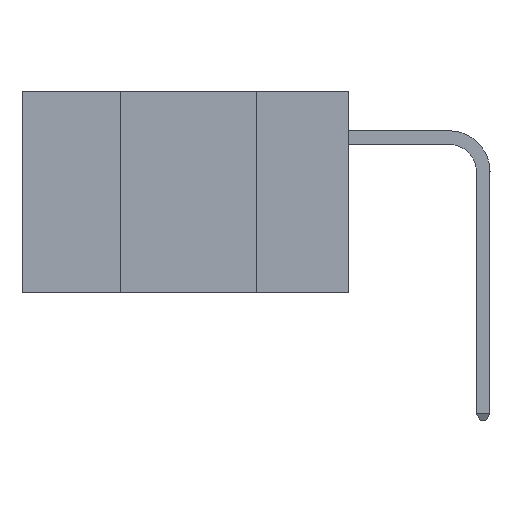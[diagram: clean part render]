
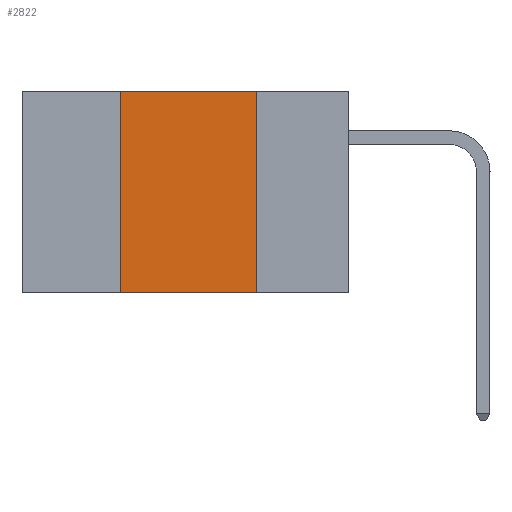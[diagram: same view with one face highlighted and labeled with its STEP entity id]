
A CAD part, left-side view. The second image highlights one B-rep face of the part: STEP entity #2822.
In plain terms, the highlighted planar face has unit normal (-1, 0, 0).
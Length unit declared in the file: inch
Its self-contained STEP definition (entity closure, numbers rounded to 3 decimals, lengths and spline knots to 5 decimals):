
#2822 = ADVANCED_FACE ( 'NONE', ( #23863 ), #23248, .F. ) ;
#2836 = DIRECTION ( 'NONE',  ( 0., 0., 1. ) ) ;
#5013 = AXIS2_PLACEMENT_3D ( 'NONE', #9218, #9372, #37027 ) ;
#6765 = CARTESIAN_POINT ( 'NONE',  ( 0., 0.42, 0. ) ) ;
#6784 = VECTOR ( 'NONE', #17891, 39.37008 ) ;
#8238 = VECTOR ( 'NONE', #37631, 39.37008 ) ;
#9218 = CARTESIAN_POINT ( 'NONE',  ( 0., 0.6, 0. ) ) ;
#9314 = LINE ( 'NONE', #23564, #8238 ) ;
#9372 = DIRECTION ( 'NONE',  ( 1., 0., 0. ) ) ;
#11196 = VERTEX_POINT ( 'NONE', #6765 ) ;
#12032 = ORIENTED_EDGE ( 'NONE', *, *, #25710, .F. ) ;
#12527 = EDGE_LOOP ( 'NONE', ( #12032, #18348, #21887, #29195 ) ) ;
#13264 = LINE ( 'NONE', #14585, #6784 ) ;
#14585 = CARTESIAN_POINT ( 'NONE',  ( 0., 0.6, 0. ) ) ;
#15386 = CARTESIAN_POINT ( 'NONE',  ( 0., 0.17, 0. ) ) ;
#16108 = CARTESIAN_POINT ( 'NONE',  ( 0., 0.42, 0. ) ) ;
#17497 = CARTESIAN_POINT ( 'NONE',  ( 0., 0.17, -0.37 ) ) ;
#17580 = LINE ( 'NONE', #16108, #38701 ) ;
#17891 = DIRECTION ( 'NONE',  ( 0., -1., 0. ) ) ;
#18348 = ORIENTED_EDGE ( 'NONE', *, *, #38684, .F. ) ;
#20844 = VERTEX_POINT ( 'NONE', #30768 ) ;
#21887 = ORIENTED_EDGE ( 'NONE', *, *, #38422, .F. ) ;
#23248 = PLANE ( 'NONE',  #5013 ) ;
#23564 = CARTESIAN_POINT ( 'NONE',  ( 0., 0.17, 0. ) ) ;
#23863 = FACE_OUTER_BOUND ( 'NONE', #12527, .T. ) ;
#25710 = EDGE_CURVE ( 'NONE', #32969, #40921, #9314, .T. ) ;
#26568 = LINE ( 'NONE', #42383, #39487 ) ;
#29195 = ORIENTED_EDGE ( 'NONE', *, *, #30340, .T. ) ;
#30340 = EDGE_CURVE ( 'NONE', #20844, #40921, #26568, .T. ) ;
#30768 = CARTESIAN_POINT ( 'NONE',  ( 0., 0.42, -0.37 ) ) ;
#32969 = VERTEX_POINT ( 'NONE', #15386 ) ;
#37027 = DIRECTION ( 'NONE',  ( 0., 0., -1. ) ) ;
#37631 = DIRECTION ( 'NONE',  ( 0., 0., -1. ) ) ;
#38422 = EDGE_CURVE ( 'NONE', #20844, #11196, #17580, .T. ) ;
#38684 = EDGE_CURVE ( 'NONE', #11196, #32969, #13264, .T. ) ;
#38701 = VECTOR ( 'NONE', #2836, 39.37008 ) ;
#39487 = VECTOR ( 'NONE', #42835, 39.37008 ) ;
#40921 = VERTEX_POINT ( 'NONE', #17497 ) ;
#42383 = CARTESIAN_POINT ( 'NONE',  ( 0., 0.6, -0.37 ) ) ;
#42835 = DIRECTION ( 'NONE',  ( 0., -1., 0. ) ) ;
